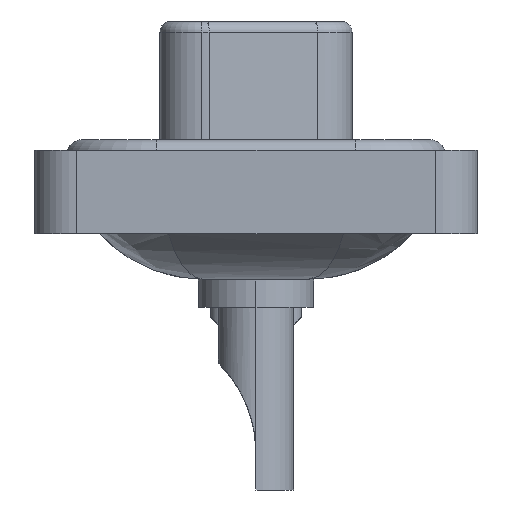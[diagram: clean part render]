
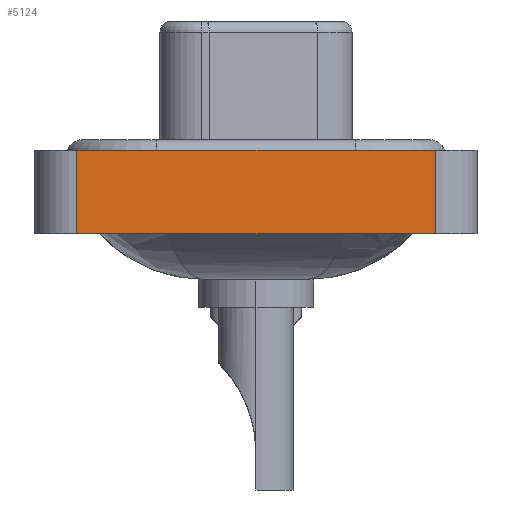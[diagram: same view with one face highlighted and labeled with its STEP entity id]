
A CAD part, left-side view. The second image highlights one B-rep face of the part: STEP entity #5124.
In plain terms, the highlighted planar face has unit normal (-1, 0, 0).
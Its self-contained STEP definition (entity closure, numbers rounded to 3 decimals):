
#213 = CARTESIAN_POINT ( 'NONE',  ( -7.35, -8.55, -3.6 ) ) ;
#1678 = CARTESIAN_POINT ( 'NONE',  ( -7.35, -8.55, -3.6 ) ) ;
#2447 = VECTOR ( 'NONE', #17775, 1000. ) ;
#3334 = DIRECTION ( 'NONE',  ( 0., 0., 1. ) ) ;
#3449 = DIRECTION ( 'NONE',  ( 0., -1., 0. ) ) ;
#4811 = VERTEX_POINT ( 'NONE', #13895 ) ;
#4934 = LINE ( 'NONE', #1678, #2447 ) ;
#5124 = ADVANCED_FACE ( 'NONE', ( #16639 ), #16872, .T. ) ;
#8555 = LINE ( 'NONE', #13718, #13469 ) ;
#9568 = ORIENTED_EDGE ( 'NONE', *, *, #12240, .F. ) ;
#10191 = LINE ( 'NONE', #23112, #15580 ) ;
#10744 = CARTESIAN_POINT ( 'NONE',  ( -7.35, -8.55, -3.6 ) ) ;
#11254 = EDGE_CURVE ( 'NONE', #18257, #18345, #4934, .T. ) ;
#11440 = VECTOR ( 'NONE', #3449, 1000. ) ;
#12240 = EDGE_CURVE ( 'NONE', #4811, #18345, #8555, .T. ) ;
#13106 = EDGE_LOOP ( 'NONE', ( #20600, #9568, #20588, #16938 ) ) ;
#13469 = VECTOR ( 'NONE', #21368, 1000. ) ;
#13718 = CARTESIAN_POINT ( 'NONE',  ( -7.35, -8.55, 0.4 ) ) ;
#13895 = CARTESIAN_POINT ( 'NONE',  ( -7.35, 8.55, 0.4 ) ) ;
#15580 = VECTOR ( 'NONE', #3334, 1000. ) ;
#16407 = EDGE_CURVE ( 'NONE', #21403, #4811, #10191, .T. ) ;
#16639 = FACE_OUTER_BOUND ( 'NONE', #13106, .T. ) ;
#16767 = DIRECTION ( 'NONE',  ( 0., 0., 1. ) ) ;
#16872 = PLANE ( 'NONE',  #16914 ) ;
#16914 = AXIS2_PLACEMENT_3D ( 'NONE', #213, #16998, #16767 ) ;
#16938 = ORIENTED_EDGE ( 'NONE', *, *, #23522, .T. ) ;
#16998 = DIRECTION ( 'NONE',  ( -1., 0., 0. ) ) ;
#17634 = CARTESIAN_POINT ( 'NONE',  ( -7.35, -8.55, -3.6 ) ) ;
#17775 = DIRECTION ( 'NONE',  ( 0., 0., 1. ) ) ;
#18257 = VERTEX_POINT ( 'NONE', #10744 ) ;
#18345 = VERTEX_POINT ( 'NONE', #20822 ) ;
#19988 = CARTESIAN_POINT ( 'NONE',  ( -7.35, 8.55, -3.6 ) ) ;
#20588 = ORIENTED_EDGE ( 'NONE', *, *, #16407, .F. ) ;
#20600 = ORIENTED_EDGE ( 'NONE', *, *, #11254, .T. ) ;
#20822 = CARTESIAN_POINT ( 'NONE',  ( -7.35, -8.55, 0.4 ) ) ;
#21368 = DIRECTION ( 'NONE',  ( 0., -1., 0. ) ) ;
#21403 = VERTEX_POINT ( 'NONE', #19988 ) ;
#21449 = LINE ( 'NONE', #17634, #11440 ) ;
#23112 = CARTESIAN_POINT ( 'NONE',  ( -7.35, 8.55, -3.6 ) ) ;
#23522 = EDGE_CURVE ( 'NONE', #21403, #18257, #21449, .T. ) ;
